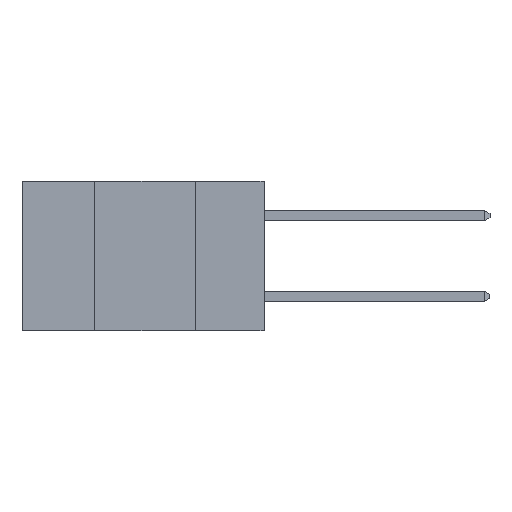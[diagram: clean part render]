
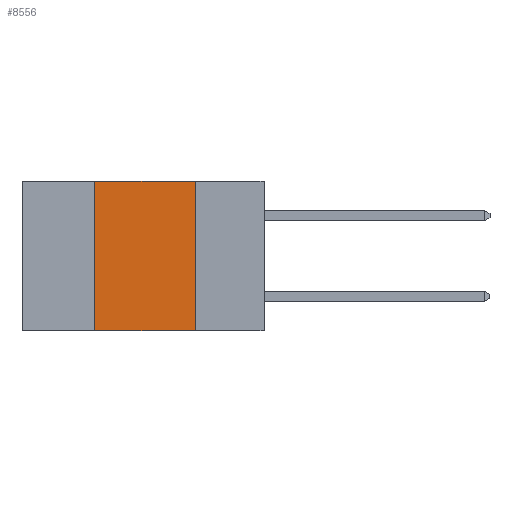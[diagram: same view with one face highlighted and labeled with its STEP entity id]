
A CAD part, left-side view. The second image highlights one B-rep face of the part: STEP entity #8556.
In plain terms, the highlighted planar face has unit normal (-1, 0, 0).
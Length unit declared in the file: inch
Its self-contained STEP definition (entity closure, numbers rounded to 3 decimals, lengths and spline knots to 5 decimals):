
#172 = VECTOR ( 'NONE', #6980, 39.37008 ) ;
#428 = VERTEX_POINT ( 'NONE', #6447 ) ;
#445 = ORIENTED_EDGE ( 'NONE', *, *, #4295, .F. ) ;
#637 = CARTESIAN_POINT ( 'NONE',  ( 0., 0.6, -0.37 ) ) ;
#717 = DIRECTION ( 'NONE',  ( 1., 0., 0. ) ) ;
#990 = VERTEX_POINT ( 'NONE', #8213 ) ;
#1296 = DIRECTION ( 'NONE',  ( 0., 0., -1. ) ) ;
#1408 = DIRECTION ( 'NONE',  ( 0., -1., 0. ) ) ;
#1486 = CARTESIAN_POINT ( 'NONE',  ( 0., 0.6, 0. ) ) ;
#1551 = CARTESIAN_POINT ( 'NONE',  ( 0., 0.6, 0. ) ) ;
#1628 = FACE_OUTER_BOUND ( 'NONE', #8283, .T. ) ;
#1988 = EDGE_CURVE ( 'NONE', #7845, #428, #5241, .T. ) ;
#2129 = CARTESIAN_POINT ( 'NONE',  ( 0., 0.17, -0.37 ) ) ;
#2327 = CARTESIAN_POINT ( 'NONE',  ( 0., 0.42, -0.37 ) ) ;
#2479 = LINE ( 'NONE', #1551, #6171 ) ;
#3932 = ORIENTED_EDGE ( 'NONE', *, *, #7837, .T. ) ;
#4295 = EDGE_CURVE ( 'NONE', #990, #7845, #2479, .T. ) ;
#4512 = VECTOR ( 'NONE', #1296, 39.37008 ) ;
#4613 = CARTESIAN_POINT ( 'NONE',  ( 0., 0.17, 0. ) ) ;
#5241 = LINE ( 'NONE', #2129, #4512 ) ;
#6013 = LINE ( 'NONE', #637, #7759 ) ;
#6171 = VECTOR ( 'NONE', #7929, 39.37008 ) ;
#6447 = CARTESIAN_POINT ( 'NONE',  ( 0., 0.17, -0.37 ) ) ;
#6980 = DIRECTION ( 'NONE',  ( 0., 0., 1. ) ) ;
#7759 = VECTOR ( 'NONE', #1408, 39.37008 ) ;
#7837 = EDGE_CURVE ( 'NONE', #8590, #428, #6013, .T. ) ;
#7845 = VERTEX_POINT ( 'NONE', #4613 ) ;
#7929 = DIRECTION ( 'NONE',  ( 0., -1., 0. ) ) ;
#8213 = CARTESIAN_POINT ( 'NONE',  ( 0., 0.42, 0. ) ) ;
#8283 = EDGE_LOOP ( 'NONE', ( #10059, #445, #8722, #3932 ) ) ;
#8556 = ADVANCED_FACE ( 'NONE', ( #1628 ), #9419, .F. ) ;
#8590 = VERTEX_POINT ( 'NONE', #8785 ) ;
#8722 = ORIENTED_EDGE ( 'NONE', *, *, #9503, .F. ) ;
#8785 = CARTESIAN_POINT ( 'NONE',  ( 0., 0.42, -0.37 ) ) ;
#8981 = LINE ( 'NONE', #2327, #172 ) ;
#9419 = PLANE ( 'NONE',  #9916 ) ;
#9503 = EDGE_CURVE ( 'NONE', #8590, #990, #8981, .T. ) ;
#9916 = AXIS2_PLACEMENT_3D ( 'NONE', #1486, #717, #10178 ) ;
#10059 = ORIENTED_EDGE ( 'NONE', *, *, #1988, .F. ) ;
#10178 = DIRECTION ( 'NONE',  ( 0., 0., -1. ) ) ;
